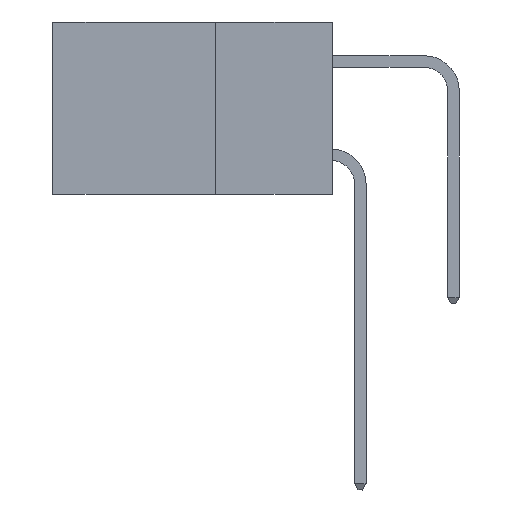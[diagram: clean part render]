
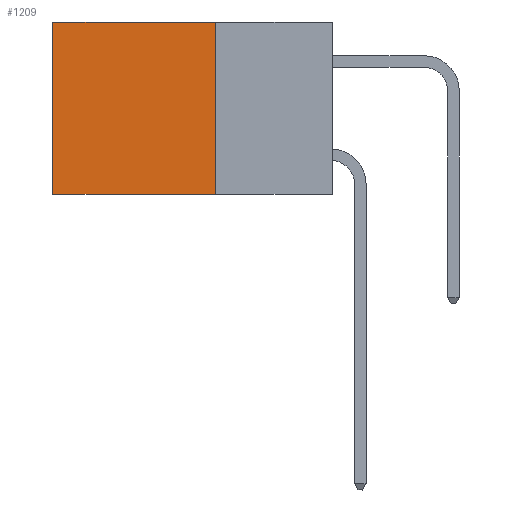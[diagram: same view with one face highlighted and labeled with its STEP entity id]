
A CAD part, left-side view. The second image highlights one B-rep face of the part: STEP entity #1209.
In plain terms, the highlighted planar face has unit normal (-1, 0, 0).
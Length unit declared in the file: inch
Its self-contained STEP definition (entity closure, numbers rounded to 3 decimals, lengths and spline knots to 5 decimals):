
#187 = DIRECTION ( 'NONE',  ( 1., 0., 0. ) ) ;
#277 = CARTESIAN_POINT ( 'NONE',  ( 0.2615, 0.25, -0.37 ) ) ;
#284 = VECTOR ( 'NONE', #1498, 39.37008 ) ;
#1190 = DIRECTION ( 'NONE',  ( 0., 0., -1. ) ) ;
#1209 = ADVANCED_FACE ( 'NONE', ( #10594 ), #1406, .F. ) ;
#1406 = PLANE ( 'NONE',  #8685 ) ;
#1498 = DIRECTION ( 'NONE',  ( 0., 1., 0. ) ) ;
#2197 = VECTOR ( 'NONE', #1190, 39.37008 ) ;
#2242 = EDGE_CURVE ( 'NONE', #11932, #12116, #14520, .T. ) ;
#2568 = ORIENTED_EDGE ( 'NONE', *, *, #4457, .T. ) ;
#2788 = VERTEX_POINT ( 'NONE', #7144 ) ;
#3417 = EDGE_CURVE ( 'NONE', #10029, #2788, #13102, .T. ) ;
#4055 = DIRECTION ( 'NONE',  ( 0., 0., -1. ) ) ;
#4457 = EDGE_CURVE ( 'NONE', #11932, #10029, #13411, .T. ) ;
#5185 = EDGE_LOOP ( 'NONE', ( #11568, #11735, #10390, #2568 ) ) ;
#5360 = CARTESIAN_POINT ( 'NONE',  ( 0.2615, 0.25, -0.37 ) ) ;
#7144 = CARTESIAN_POINT ( 'NONE',  ( 0.2615, 0.6, -0.37 ) ) ;
#7883 = LINE ( 'NONE', #7967, #12341 ) ;
#7967 = CARTESIAN_POINT ( 'NONE',  ( 0.2615, 0.25, -0.37 ) ) ;
#8685 = AXIS2_PLACEMENT_3D ( 'NONE', #277, #187, #15933 ) ;
#8733 = CARTESIAN_POINT ( 'NONE',  ( 0.2615, 0.6, 0. ) ) ;
#9054 = VECTOR ( 'NONE', #4055, 39.37008 ) ;
#9139 = CARTESIAN_POINT ( 'NONE',  ( 0.2615, 0.25, 0. ) ) ;
#10029 = VERTEX_POINT ( 'NONE', #8733 ) ;
#10390 = ORIENTED_EDGE ( 'NONE', *, *, #2242, .F. ) ;
#10405 = CARTESIAN_POINT ( 'NONE',  ( 0.2615, 0.25, 0. ) ) ;
#10594 = FACE_OUTER_BOUND ( 'NONE', #5185, .T. ) ;
#11568 = ORIENTED_EDGE ( 'NONE', *, *, #3417, .T. ) ;
#11678 = CARTESIAN_POINT ( 'NONE',  ( 0.2615, 0.6, -0.37 ) ) ;
#11735 = ORIENTED_EDGE ( 'NONE', *, *, #16398, .F. ) ;
#11932 = VERTEX_POINT ( 'NONE', #10405 ) ;
#11933 = DIRECTION ( 'NONE',  ( 0., 1., 0. ) ) ;
#12116 = VERTEX_POINT ( 'NONE', #12226 ) ;
#12226 = CARTESIAN_POINT ( 'NONE',  ( 0.2615, 0.25, -0.37 ) ) ;
#12341 = VECTOR ( 'NONE', #11933, 39.37008 ) ;
#13102 = LINE ( 'NONE', #11678, #2197 ) ;
#13411 = LINE ( 'NONE', #9139, #284 ) ;
#14520 = LINE ( 'NONE', #5360, #9054 ) ;
#15933 = DIRECTION ( 'NONE',  ( 0., 0., -1. ) ) ;
#16398 = EDGE_CURVE ( 'NONE', #12116, #2788, #7883, .T. ) ;
